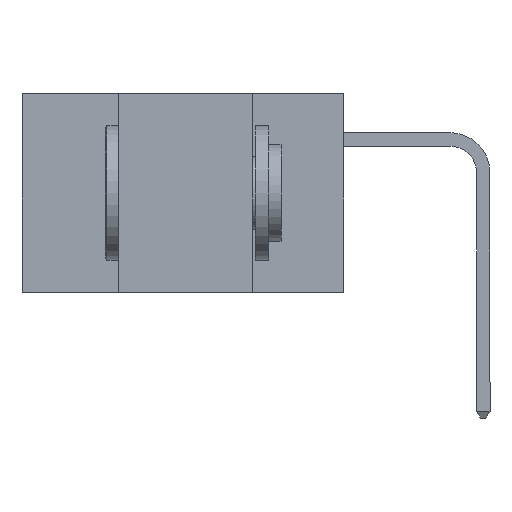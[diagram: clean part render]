
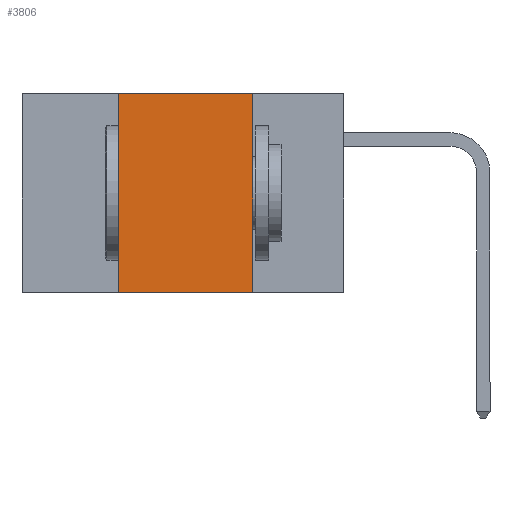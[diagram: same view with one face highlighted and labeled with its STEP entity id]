
A CAD part, left-side view. The second image highlights one B-rep face of the part: STEP entity #3806.
In plain terms, the highlighted planar face has unit normal (-1, 0, 0).
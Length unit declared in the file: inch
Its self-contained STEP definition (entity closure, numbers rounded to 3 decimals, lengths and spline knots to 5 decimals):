
#12 = VECTOR ( 'NONE', #12484, 39.37008 ) ;
#549 = ORIENTED_EDGE ( 'NONE', *, *, #7507, .T. ) ;
#1445 = CARTESIAN_POINT ( 'NONE',  ( 0., 0.6, 0. ) ) ;
#2058 = CARTESIAN_POINT ( 'NONE',  ( 0., 0.17, -0.37 ) ) ;
#2205 = VECTOR ( 'NONE', #9735, 39.37008 ) ;
#2383 = CARTESIAN_POINT ( 'NONE',  ( 0., 0.6, 0. ) ) ;
#2666 = FACE_OUTER_BOUND ( 'NONE', #15039, .T. ) ;
#3066 = DIRECTION ( 'NONE',  ( 0., 0., -1. ) ) ;
#3197 = LINE ( 'NONE', #7303, #12477 ) ;
#3525 = ORIENTED_EDGE ( 'NONE', *, *, #7923, .F. ) ;
#3655 = DIRECTION ( 'NONE',  ( 1., 0., 0. ) ) ;
#3806 = ADVANCED_FACE ( 'NONE', ( #2666 ), #14002, .F. ) ;
#4211 = CARTESIAN_POINT ( 'NONE',  ( 0., 0.17, 0. ) ) ;
#5270 = CARTESIAN_POINT ( 'NONE',  ( 0., 0.42, -0.37 ) ) ;
#5528 = LINE ( 'NONE', #14422, #14842 ) ;
#6762 = LINE ( 'NONE', #11315, #12 ) ;
#7303 = CARTESIAN_POINT ( 'NONE',  ( 0., 0.42, 0. ) ) ;
#7507 = EDGE_CURVE ( 'NONE', #12589, #10689, #6762, .T. ) ;
#7923 = EDGE_CURVE ( 'NONE', #14135, #15523, #12277, .T. ) ;
#8305 = EDGE_CURVE ( 'NONE', #12589, #14135, #3197, .T. ) ;
#8500 = DIRECTION ( 'NONE',  ( 0., 0., 1. ) ) ;
#9120 = EDGE_CURVE ( 'NONE', #15523, #10689, #5528, .T. ) ;
#9735 = DIRECTION ( 'NONE',  ( 0., -1., 0. ) ) ;
#10689 = VERTEX_POINT ( 'NONE', #2058 ) ;
#11315 = CARTESIAN_POINT ( 'NONE',  ( 0., 0.6, -0.37 ) ) ;
#12277 = LINE ( 'NONE', #2383, #2205 ) ;
#12477 = VECTOR ( 'NONE', #8500, 39.37008 ) ;
#12484 = DIRECTION ( 'NONE',  ( 0., -1., 0. ) ) ;
#12589 = VERTEX_POINT ( 'NONE', #5270 ) ;
#12787 = ORIENTED_EDGE ( 'NONE', *, *, #9120, .F. ) ;
#13142 = ORIENTED_EDGE ( 'NONE', *, *, #8305, .F. ) ;
#13833 = AXIS2_PLACEMENT_3D ( 'NONE', #1445, #3655, #3066 ) ;
#14002 = PLANE ( 'NONE',  #13833 ) ;
#14135 = VERTEX_POINT ( 'NONE', #14871 ) ;
#14422 = CARTESIAN_POINT ( 'NONE',  ( 0., 0.17, 0. ) ) ;
#14842 = VECTOR ( 'NONE', #15512, 39.37008 ) ;
#14871 = CARTESIAN_POINT ( 'NONE',  ( 0., 0.42, 0. ) ) ;
#15039 = EDGE_LOOP ( 'NONE', ( #12787, #3525, #13142, #549 ) ) ;
#15512 = DIRECTION ( 'NONE',  ( 0., 0., -1. ) ) ;
#15523 = VERTEX_POINT ( 'NONE', #4211 ) ;
